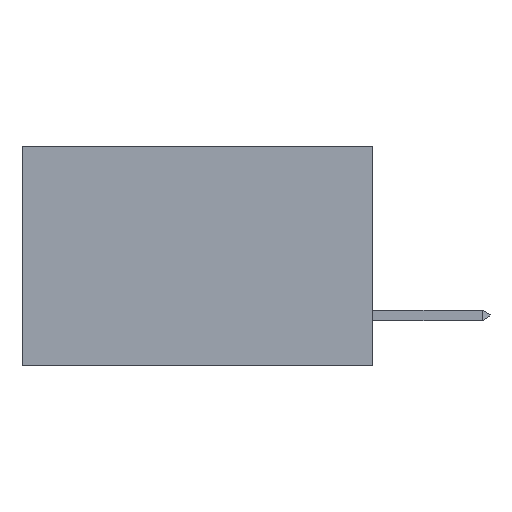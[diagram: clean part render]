
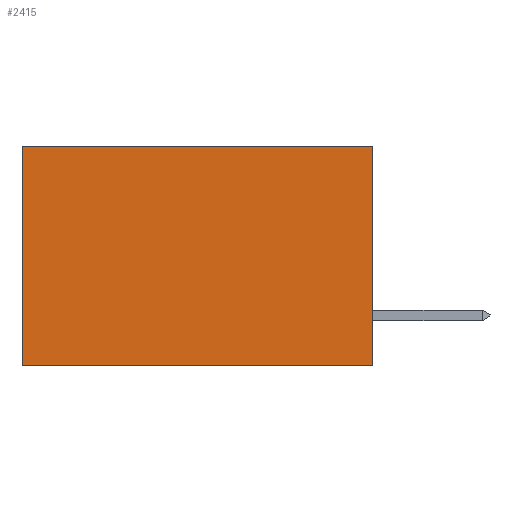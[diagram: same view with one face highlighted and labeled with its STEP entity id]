
A CAD part, left-side view. The second image highlights one B-rep face of the part: STEP entity #2415.
In plain terms, the highlighted planar face has unit normal (-1, 0, 0).
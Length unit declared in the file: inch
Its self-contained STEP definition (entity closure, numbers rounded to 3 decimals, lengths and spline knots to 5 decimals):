
#68 = CARTESIAN_POINT ( 'NONE',  ( 0.277, 0., -0.37 ) ) ;
#560 = EDGE_CURVE ( 'NONE', #14116, #12735, #5267, .T. ) ;
#697 = EDGE_LOOP ( 'NONE', ( #2218, #12062, #6144, #9296 ) ) ;
#1254 = EDGE_CURVE ( 'NONE', #12000, #12995, #11110, .T. ) ;
#2218 = ORIENTED_EDGE ( 'NONE', *, *, #14519, .T. ) ;
#2415 = ADVANCED_FACE ( 'NONE', ( #10020 ), #10013, .F. ) ;
#2683 = CARTESIAN_POINT ( 'NONE',  ( 0.277, 0., -0.37 ) ) ;
#3877 = DIRECTION ( 'NONE',  ( 0., 0., -1. ) ) ;
#4125 = CARTESIAN_POINT ( 'NONE',  ( 0.277, 0.59, -0.37 ) ) ;
#4822 = VECTOR ( 'NONE', #3877, 39.37008 ) ;
#4895 = CARTESIAN_POINT ( 'NONE',  ( 0.277, 0.59, 0. ) ) ;
#5267 = LINE ( 'NONE', #6921, #14177 ) ;
#5664 = CARTESIAN_POINT ( 'NONE',  ( 0.277, 0.59, -0.37 ) ) ;
#5715 = DIRECTION ( 'NONE',  ( 0., 0., -1. ) ) ;
#6144 = ORIENTED_EDGE ( 'NONE', *, *, #14159, .F. ) ;
#6921 = CARTESIAN_POINT ( 'NONE',  ( 0.277, 0., 0. ) ) ;
#8013 = VECTOR ( 'NONE', #8771, 39.37008 ) ;
#8172 = VECTOR ( 'NONE', #5715, 39.37008 ) ;
#8285 = DIRECTION ( 'NONE',  ( 0., 1., 0. ) ) ;
#8771 = DIRECTION ( 'NONE',  ( 0., 1., 0. ) ) ;
#9296 = ORIENTED_EDGE ( 'NONE', *, *, #560, .T. ) ;
#9799 = DIRECTION ( 'NONE',  ( 0., 0., -1. ) ) ;
#9826 = DIRECTION ( 'NONE',  ( 1., 0., 0. ) ) ;
#10013 = PLANE ( 'NONE',  #12405 ) ;
#10020 = FACE_OUTER_BOUND ( 'NONE', #697, .T. ) ;
#10168 = CARTESIAN_POINT ( 'NONE',  ( 0.277, 0., -0.37 ) ) ;
#11110 = LINE ( 'NONE', #14053, #8013 ) ;
#12000 = VERTEX_POINT ( 'NONE', #68 ) ;
#12010 = CARTESIAN_POINT ( 'NONE',  ( 0.277, 0., 0. ) ) ;
#12062 = ORIENTED_EDGE ( 'NONE', *, *, #1254, .F. ) ;
#12405 = AXIS2_PLACEMENT_3D ( 'NONE', #10168, #9826, #9799 ) ;
#12735 = VERTEX_POINT ( 'NONE', #4895 ) ;
#12995 = VERTEX_POINT ( 'NONE', #4125 ) ;
#14053 = CARTESIAN_POINT ( 'NONE',  ( 0.277, 0., -0.37 ) ) ;
#14116 = VERTEX_POINT ( 'NONE', #12010 ) ;
#14159 = EDGE_CURVE ( 'NONE', #14116, #12000, #14809, .T. ) ;
#14177 = VECTOR ( 'NONE', #8285, 39.37008 ) ;
#14302 = LINE ( 'NONE', #5664, #8172 ) ;
#14519 = EDGE_CURVE ( 'NONE', #12735, #12995, #14302, .T. ) ;
#14809 = LINE ( 'NONE', #2683, #4822 ) ;
